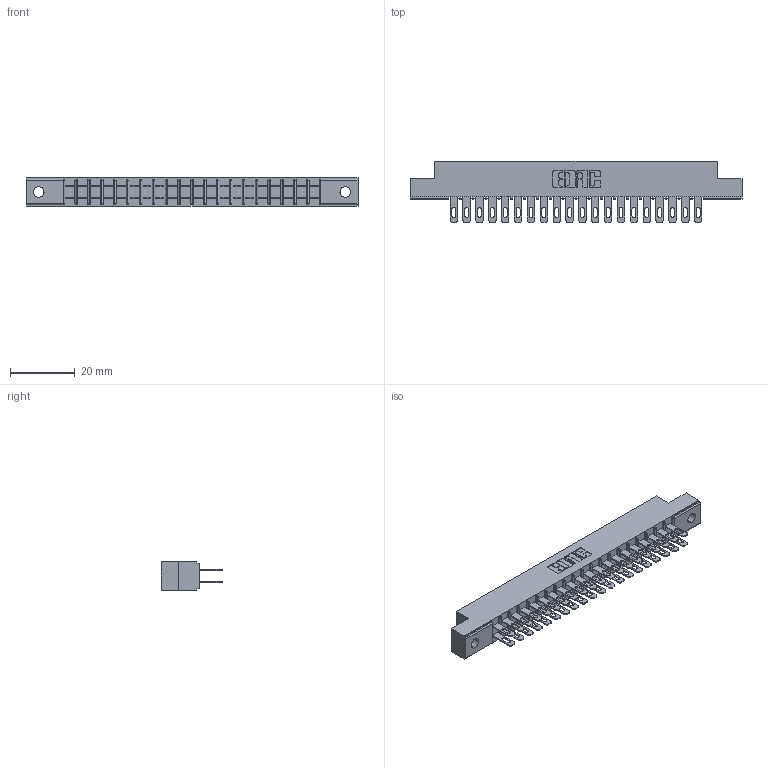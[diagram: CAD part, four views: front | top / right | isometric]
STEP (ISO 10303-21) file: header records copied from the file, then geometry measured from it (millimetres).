
FILE_DESCRIPTION (( 'STEP AP203' ), '1' );
FILE_NAME ('305-040-500-202.STEP', '2019-09-09T18:46:46', ( '' ), ( '' ), 'SwSTEP 2.0', 'SolidWorks 2016', '' );
FILE_SCHEMA (( 'CONFIG_CONTROL_DESIGN' ));
Length unit declared in the file: inch
Products named in the file (3): 305 Part_.128 Dia; 305-040-500-202; 305-290-001_500
Assembly tree (41 placements, depth 2):
  305-040-500-202
    305 Part_.128 Dia
    305-290-001_500  x40
Bounding box: 102.26 x 18.85 x 8.71 mm (x, y, z)
Volume: 6499.3 mm3; surface area: 12620.3 mm2
Topology: 41 solids, 41 shells, 2116 faces, 6056 edges, 3928 vertices
Faces by surface type: plane 1188, cylinder 848, sphere 80
Entity records: 24357 total; most frequent: CARTESIAN_POINT 4030, ORIENTED_EDGE 3996, DIRECTION 3918, EDGE_CURVE 1998, LINE 1590, VECTOR 1590, VERTEX_POINT 1276, AXIS2_PLACEMENT_3D 1164
